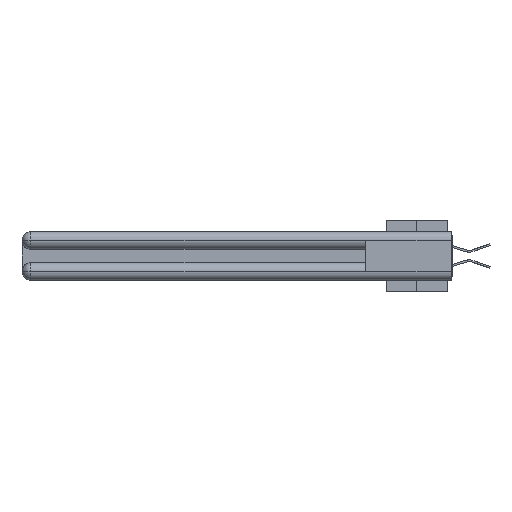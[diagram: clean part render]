
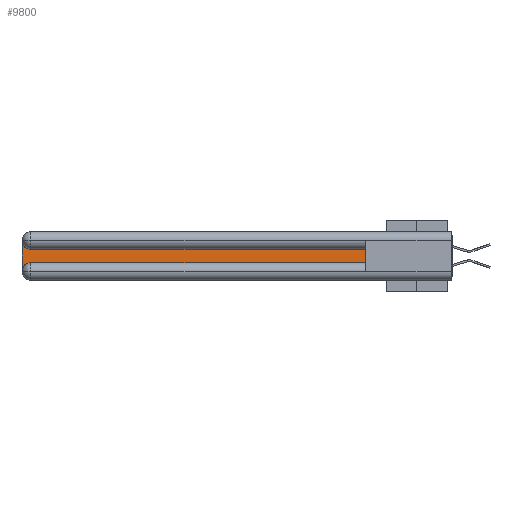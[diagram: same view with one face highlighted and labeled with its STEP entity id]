
A CAD part, left-side view. The second image highlights one B-rep face of the part: STEP entity #9800.
In plain terms, the highlighted planar face has unit normal (-1, 0, 0).
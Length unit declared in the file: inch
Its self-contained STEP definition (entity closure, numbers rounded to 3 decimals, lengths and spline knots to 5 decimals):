
#1690 = LINE ( 'NONE', #19586, #40733 ) ;
#1898 = CARTESIAN_POINT ( 'NONE',  ( 0.075, 2.94, -0.0625 ) ) ;
#2675 = DIRECTION ( 'NONE',  ( 0., 0., -1. ) ) ;
#4332 = CARTESIAN_POINT ( 'NONE',  ( 0.075, 0.6, -0.1225 ) ) ;
#5035 = CARTESIAN_POINT ( 'NONE',  ( 0.075, 0.6, -0.2175 ) ) ;
#5387 = VERTEX_POINT ( 'NONE', #5035 ) ;
#8393 = DIRECTION ( 'NONE',  ( 0., 0., -1. ) ) ;
#9408 = CIRCLE ( 'NONE', #25233, 0.06 ) ;
#9800 = ADVANCED_FACE ( 'NONE', ( #15818 ), #28265, .F. ) ;
#10237 = VERTEX_POINT ( 'NONE', #17228 ) ;
#10359 = VERTEX_POINT ( 'NONE', #11812 ) ;
#11392 = CARTESIAN_POINT ( 'NONE',  ( 0.075, 0.6, -0.2175 ) ) ;
#11812 = CARTESIAN_POINT ( 'NONE',  ( 0.075, 2.94, -0.2175 ) ) ;
#11859 = CARTESIAN_POINT ( 'NONE',  ( 0.075, 3., -0.1225 ) ) ;
#14282 = VERTEX_POINT ( 'NONE', #39276 ) ;
#14493 = VECTOR ( 'NONE', #31565, 39.37008 ) ;
#14801 = EDGE_CURVE ( 'NONE', #14282, #34046, #39297, .T. ) ;
#14982 = CARTESIAN_POINT ( 'NONE',  ( 0.075, 2.94, -0.2775 ) ) ;
#15118 = DIRECTION ( 'NONE',  ( 1., 0., 0. ) ) ;
#15818 = FACE_OUTER_BOUND ( 'NONE', #23757, .T. ) ;
#17228 = CARTESIAN_POINT ( 'NONE',  ( 0.075, 3., -0.0625 ) ) ;
#17665 = LINE ( 'NONE', #26707, #31847 ) ;
#18142 = DIRECTION ( 'NONE',  ( 1., 0., 0. ) ) ;
#19586 = CARTESIAN_POINT ( 'NONE',  ( 0.075, 3., -0.2175 ) ) ;
#20167 = EDGE_CURVE ( 'NONE', #10237, #29306, #1690, .T. ) ;
#20953 = VECTOR ( 'NONE', #23301, 39.37008 ) ;
#21730 = DIRECTION ( 'NONE',  ( 1., 0., 0. ) ) ;
#22842 = ORIENTED_EDGE ( 'NONE', *, *, #29508, .T. ) ;
#23180 = DIRECTION ( 'NONE',  ( 0., 0., 1. ) ) ;
#23301 = DIRECTION ( 'NONE',  ( 0., 1., 0. ) ) ;
#23757 = EDGE_LOOP ( 'NONE', ( #40599, #31152, #25496, #23932, #32503, #22842 ) ) ;
#23932 = ORIENTED_EDGE ( 'NONE', *, *, #25115, .T. ) ;
#25115 = EDGE_CURVE ( 'NONE', #29306, #10359, #9408, .T. ) ;
#25233 = AXIS2_PLACEMENT_3D ( 'NONE', #14982, #15118, #40950 ) ;
#25374 = EDGE_CURVE ( 'NONE', #10359, #5387, #31691, .T. ) ;
#25496 = ORIENTED_EDGE ( 'NONE', *, *, #20167, .T. ) ;
#25927 = AXIS2_PLACEMENT_3D ( 'NONE', #1898, #18142, #8393 ) ;
#26707 = CARTESIAN_POINT ( 'NONE',  ( 0.075, 0.6, -0.2175 ) ) ;
#26756 = CIRCLE ( 'NONE', #25927, 0.06 ) ;
#28265 = PLANE ( 'NONE',  #32606 ) ;
#29306 = VERTEX_POINT ( 'NONE', #35000 ) ;
#29508 = EDGE_CURVE ( 'NONE', #5387, #14282, #17665, .T. ) ;
#29687 = EDGE_CURVE ( 'NONE', #34046, #10237, #26756, .T. ) ;
#31152 = ORIENTED_EDGE ( 'NONE', *, *, #29687, .T. ) ;
#31565 = DIRECTION ( 'NONE',  ( 0., -1., 0. ) ) ;
#31691 = LINE ( 'NONE', #11392, #14493 ) ;
#31847 = VECTOR ( 'NONE', #23180, 39.37008 ) ;
#32503 = ORIENTED_EDGE ( 'NONE', *, *, #25374, .T. ) ;
#32606 = AXIS2_PLACEMENT_3D ( 'NONE', #11859, #21730, #2675 ) ;
#34046 = VERTEX_POINT ( 'NONE', #36575 ) ;
#35000 = CARTESIAN_POINT ( 'NONE',  ( 0.075, 3., -0.2775 ) ) ;
#36575 = CARTESIAN_POINT ( 'NONE',  ( 0.075, 2.94, -0.1225 ) ) ;
#39198 = DIRECTION ( 'NONE',  ( 0., 0., -1. ) ) ;
#39276 = CARTESIAN_POINT ( 'NONE',  ( 0.075, 0.6, -0.1225 ) ) ;
#39297 = LINE ( 'NONE', #4332, #20953 ) ;
#40599 = ORIENTED_EDGE ( 'NONE', *, *, #14801, .T. ) ;
#40733 = VECTOR ( 'NONE', #39198, 39.37008 ) ;
#40950 = DIRECTION ( 'NONE',  ( 0., 0., -1. ) ) ;
